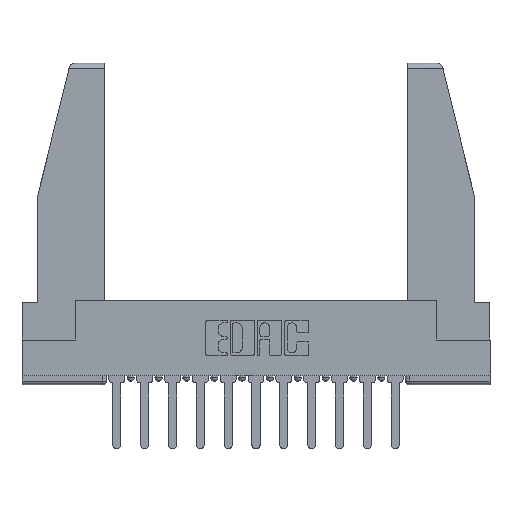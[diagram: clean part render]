
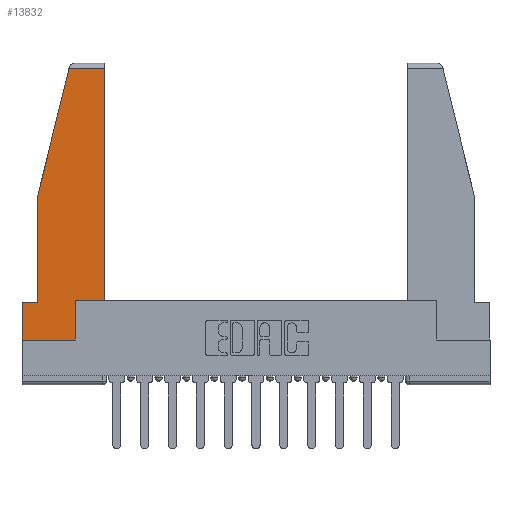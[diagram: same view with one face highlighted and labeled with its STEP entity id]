
A CAD part, top view. The second image highlights one B-rep face of the part: STEP entity #13832.
In plain terms, the highlighted planar face has unit normal (0, 0, 1).
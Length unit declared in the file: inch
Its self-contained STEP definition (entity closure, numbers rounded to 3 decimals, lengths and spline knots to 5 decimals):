
#37 = EDGE_LOOP ( 'NONE', ( #8138, #3919, #9607, #14918, #6302, #13757, #4039, #4156, #7666 ) ) ;
#186 = CARTESIAN_POINT ( 'NONE',  ( 0.461, 0.223, 0. ) ) ;
#338 = AXIS2_PLACEMENT_3D ( 'NONE', #3758, #2504, #9759 ) ;
#509 = FACE_OUTER_BOUND ( 'NONE', #37, .T. ) ;
#1022 = VECTOR ( 'NONE', #1477, 39.37008 ) ;
#1173 = DIRECTION ( 'NONE',  ( 0., -1., 0. ) ) ;
#1452 = LINE ( 'NONE', #7690, #7695 ) ;
#1477 = DIRECTION ( 'NONE',  ( 0., 1., 0. ) ) ;
#1582 = EDGE_CURVE ( 'NONE', #2539, #11603, #11859, .T. ) ;
#1885 = VERTEX_POINT ( 'NONE', #2976 ) ;
#2015 = CARTESIAN_POINT ( 'NONE',  ( 0., 0., 0. ) ) ;
#2260 = EDGE_CURVE ( 'NONE', #11603, #9845, #5137, .T. ) ;
#2421 = LINE ( 'NONE', #15869, #5587 ) ;
#2504 = DIRECTION ( 'NONE',  ( 0., 0., 1. ) ) ;
#2517 = VECTOR ( 'NONE', #5173, 39.37008 ) ;
#2539 = VERTEX_POINT ( 'NONE', #9017 ) ;
#2760 = VERTEX_POINT ( 'NONE', #14168 ) ;
#2896 = VERTEX_POINT ( 'NONE', #8411 ) ;
#2976 = CARTESIAN_POINT ( 'NONE',  ( 0.461, 1.52, 0. ) ) ;
#3469 = CARTESIAN_POINT ( 'NONE',  ( 0., 0.21, 0. ) ) ;
#3700 = PLANE ( 'NONE',  #338 ) ;
#3758 = CARTESIAN_POINT ( 'NONE',  ( 0., 0., 0. ) ) ;
#3866 = CARTESIAN_POINT ( 'NONE',  ( 0.086, 0.8, 0. ) ) ;
#3919 = ORIENTED_EDGE ( 'NONE', *, *, #3955, .T. ) ;
#3955 = EDGE_CURVE ( 'NONE', #1885, #7431, #5847, .T. ) ;
#4007 = CARTESIAN_POINT ( 'NONE',  ( 0.297, 0., 0. ) ) ;
#4039 = ORIENTED_EDGE ( 'NONE', *, *, #10823, .T. ) ;
#4156 = ORIENTED_EDGE ( 'NONE', *, *, #1582, .T. ) ;
#5137 = LINE ( 'NONE', #13526, #13578 ) ;
#5173 = DIRECTION ( 'NONE',  ( -1., 0., 0. ) ) ;
#5508 = EDGE_CURVE ( 'NONE', #9845, #1885, #8483, .T. ) ;
#5587 = VECTOR ( 'NONE', #11985, 39.37008 ) ;
#5847 = LINE ( 'NONE', #12510, #2517 ) ;
#6099 = VERTEX_POINT ( 'NONE', #6466 ) ;
#6302 = ORIENTED_EDGE ( 'NONE', *, *, #6701, .T. ) ;
#6466 = CARTESIAN_POINT ( 'NONE',  ( 0., 0., 0. ) ) ;
#6701 = EDGE_CURVE ( 'NONE', #2760, #13252, #1452, .T. ) ;
#7229 = CARTESIAN_POINT ( 'NONE',  ( 0.297, 0.223, 0. ) ) ;
#7424 = DIRECTION ( 'NONE',  ( 1., 0., 0. ) ) ;
#7431 = VERTEX_POINT ( 'NONE', #8182 ) ;
#7666 = ORIENTED_EDGE ( 'NONE', *, *, #2260, .T. ) ;
#7690 = CARTESIAN_POINT ( 'NONE',  ( 0., 0.21, 0. ) ) ;
#7695 = VECTOR ( 'NONE', #7854, 39.37008 ) ;
#7838 = DIRECTION ( 'NONE',  ( 0., 1., 0. ) ) ;
#7854 = DIRECTION ( 'NONE',  ( -1., 0., 0. ) ) ;
#8138 = ORIENTED_EDGE ( 'NONE', *, *, #5508, .T. ) ;
#8182 = CARTESIAN_POINT ( 'NONE',  ( 0.2636, 1.52, 0. ) ) ;
#8411 = CARTESIAN_POINT ( 'NONE',  ( 0.086, 0.8, 0. ) ) ;
#8483 = LINE ( 'NONE', #11629, #13657 ) ;
#8485 = VECTOR ( 'NONE', #15885, 39.37008 ) ;
#8866 = EDGE_CURVE ( 'NONE', #7431, #2896, #2421, .T. ) ;
#9017 = CARTESIAN_POINT ( 'NONE',  ( 0.297, 0., 0. ) ) ;
#9318 = EDGE_CURVE ( 'NONE', #2896, #2760, #13039, .T. ) ;
#9607 = ORIENTED_EDGE ( 'NONE', *, *, #8866, .T. ) ;
#9759 = DIRECTION ( 'NONE',  ( 1., 0., 0. ) ) ;
#9845 = VERTEX_POINT ( 'NONE', #186 ) ;
#10823 = EDGE_CURVE ( 'NONE', #6099, #2539, #13559, .T. ) ;
#11603 = VERTEX_POINT ( 'NONE', #7229 ) ;
#11629 = CARTESIAN_POINT ( 'NONE',  ( 0.461, 0.223, 0. ) ) ;
#11859 = LINE ( 'NONE', #4007, #1022 ) ;
#11985 = DIRECTION ( 'NONE',  ( -0.239, -0.971, 0. ) ) ;
#12510 = CARTESIAN_POINT ( 'NONE',  ( 0., 1.52, 0. ) ) ;
#12684 = LINE ( 'NONE', #15778, #8485 ) ;
#13039 = LINE ( 'NONE', #3866, #15744 ) ;
#13218 = DIRECTION ( 'NONE',  ( 1., 0., 0. ) ) ;
#13252 = VERTEX_POINT ( 'NONE', #3469 ) ;
#13526 = CARTESIAN_POINT ( 'NONE',  ( 0.297, 0.223, 0. ) ) ;
#13559 = LINE ( 'NONE', #2015, #15692 ) ;
#13578 = VECTOR ( 'NONE', #7424, 39.37008 ) ;
#13657 = VECTOR ( 'NONE', #7838, 39.37008 ) ;
#13757 = ORIENTED_EDGE ( 'NONE', *, *, #14529, .T. ) ;
#13832 = ADVANCED_FACE ( 'NONE', ( #509 ), #3700, .T. ) ;
#14168 = CARTESIAN_POINT ( 'NONE',  ( 0.086, 0.21, 0. ) ) ;
#14529 = EDGE_CURVE ( 'NONE', #13252, #6099, #12684, .T. ) ;
#14918 = ORIENTED_EDGE ( 'NONE', *, *, #9318, .T. ) ;
#15692 = VECTOR ( 'NONE', #13218, 39.37008 ) ;
#15744 = VECTOR ( 'NONE', #1173, 39.37008 ) ;
#15778 = CARTESIAN_POINT ( 'NONE',  ( 0., 0.21, 0. ) ) ;
#15869 = CARTESIAN_POINT ( 'NONE',  ( 0.271, 1.55, 0. ) ) ;
#15885 = DIRECTION ( 'NONE',  ( 0., -1., 0. ) ) ;
